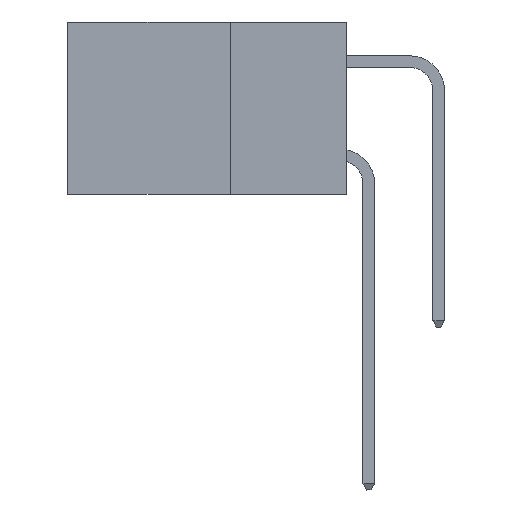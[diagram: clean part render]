
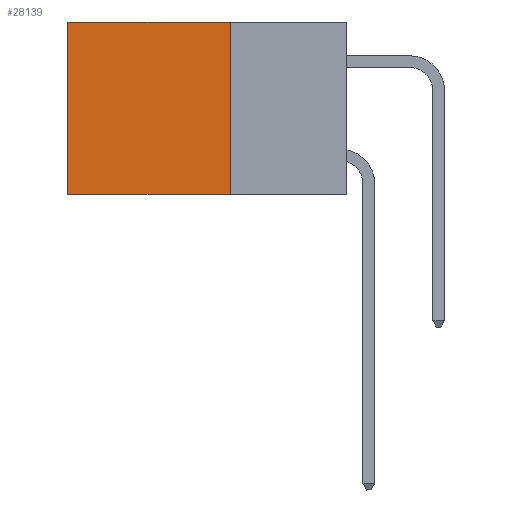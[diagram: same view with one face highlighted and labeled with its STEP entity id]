
A CAD part, left-side view. The second image highlights one B-rep face of the part: STEP entity #28139.
In plain terms, the highlighted planar face has unit normal (-1, 0, 0).
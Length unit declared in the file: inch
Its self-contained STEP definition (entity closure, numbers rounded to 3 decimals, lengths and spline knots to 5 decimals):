
#1156 = EDGE_CURVE ( 'NONE', #42605, #31375, #3537, .T. ) ;
#1589 = ORIENTED_EDGE ( 'NONE', *, *, #33201, .T. ) ;
#2768 = CARTESIAN_POINT ( 'NONE',  ( 0.2875, 0.25, -0.37 ) ) ;
#3537 = LINE ( 'NONE', #26819, #29491 ) ;
#5346 = ORIENTED_EDGE ( 'NONE', *, *, #9225, .F. ) ;
#6041 = VECTOR ( 'NONE', #18551, 39.37008 ) ;
#9225 = EDGE_CURVE ( 'NONE', #31375, #12695, #42417, .T. ) ;
#10123 = EDGE_CURVE ( 'NONE', #11290, #12695, #15565, .T. ) ;
#10812 = ORIENTED_EDGE ( 'NONE', *, *, #10123, .T. ) ;
#11290 = VERTEX_POINT ( 'NONE', #13995 ) ;
#11821 = CARTESIAN_POINT ( 'NONE',  ( 0.2875, 0.25, 0. ) ) ;
#12695 = VERTEX_POINT ( 'NONE', #14465 ) ;
#13995 = CARTESIAN_POINT ( 'NONE',  ( 0.2875, 0.6, 0. ) ) ;
#14465 = CARTESIAN_POINT ( 'NONE',  ( 0.2875, 0.6, -0.37 ) ) ;
#15565 = LINE ( 'NONE', #38001, #32422 ) ;
#15649 = VECTOR ( 'NONE', #40919, 39.37008 ) ;
#18551 = DIRECTION ( 'NONE',  ( 0., 1., 0. ) ) ;
#18984 = DIRECTION ( 'NONE',  ( 1., 0., 0. ) ) ;
#22658 = EDGE_LOOP ( 'NONE', ( #10812, #5346, #32642, #1589 ) ) ;
#24139 = LINE ( 'NONE', #11821, #6041 ) ;
#26304 = FACE_OUTER_BOUND ( 'NONE', #22658, .T. ) ;
#26819 = CARTESIAN_POINT ( 'NONE',  ( 0.2875, 0.25, 0. ) ) ;
#28050 = AXIS2_PLACEMENT_3D ( 'NONE', #35689, #18984, #42404 ) ;
#28139 = ADVANCED_FACE ( 'NONE', ( #26304 ), #32339, .F. ) ;
#29491 = VECTOR ( 'NONE', #30164, 39.37008 ) ;
#30164 = DIRECTION ( 'NONE',  ( 0., 0., -1. ) ) ;
#31375 = VERTEX_POINT ( 'NONE', #2768 ) ;
#32339 = PLANE ( 'NONE',  #28050 ) ;
#32422 = VECTOR ( 'NONE', #41380, 39.37008 ) ;
#32642 = ORIENTED_EDGE ( 'NONE', *, *, #1156, .F. ) ;
#33201 = EDGE_CURVE ( 'NONE', #42605, #11290, #24139, .T. ) ;
#35689 = CARTESIAN_POINT ( 'NONE',  ( 0.2875, 0.25, 0. ) ) ;
#37538 = CARTESIAN_POINT ( 'NONE',  ( 0.2875, 0.25, -0.37 ) ) ;
#38001 = CARTESIAN_POINT ( 'NONE',  ( 0.2875, 0.6, 0. ) ) ;
#40919 = DIRECTION ( 'NONE',  ( 0., 1., 0. ) ) ;
#41158 = CARTESIAN_POINT ( 'NONE',  ( 0.2875, 0.25, 0. ) ) ;
#41380 = DIRECTION ( 'NONE',  ( 0., 0., -1. ) ) ;
#42404 = DIRECTION ( 'NONE',  ( 0., 0., -1. ) ) ;
#42417 = LINE ( 'NONE', #37538, #15649 ) ;
#42605 = VERTEX_POINT ( 'NONE', #41158 ) ;
